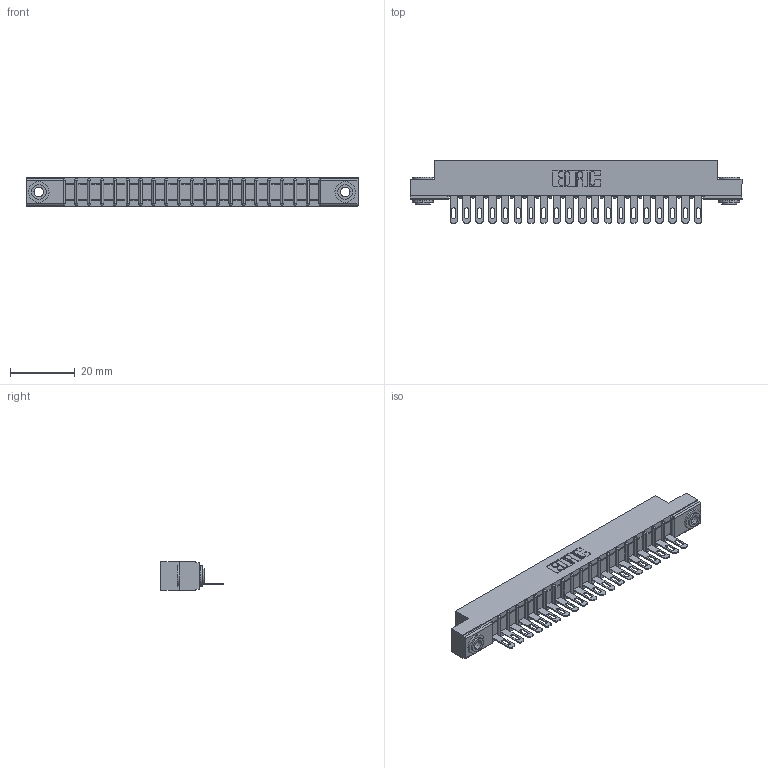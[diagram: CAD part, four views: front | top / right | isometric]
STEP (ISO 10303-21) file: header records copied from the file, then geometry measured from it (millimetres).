
FILE_DESCRIPTION (( 'STEP AP203' ), '1' );
FILE_NAME ('307-020-505-103.STEP', '2019-09-03T18:37:47', ( '' ), ( '' ), 'SwSTEP 2.0', 'SolidWorks 2016', '' );
FILE_SCHEMA (( 'CONFIG_CONTROL_DESIGN' ));
Length unit declared in the file: inch
Products named in the file (4): 345-250-002_345-250-002-102; 307 Part_.156 Dia Mounting Holes; 307-290-001_505; 307-020-505-103
Assembly tree (23 placements, depth 2):
  307-020-505-103
    307 Part_.156 Dia Mounting Holes
    307-290-001_505  x20
    345-250-002_345-250-002-102  x2
Bounding box: 102.26 x 19.18 x 8.71 mm (x, y, z)
Volume: 6489.7 mm3; surface area: 10400.1 mm2
Topology: 23 solids, 23 shells, 1311 faces, 3675 edges, 2362 vertices
Faces by surface type: plane 814, cylinder 447, sphere 42, cone 8
Entity records: 20897 total; most frequent: CARTESIAN_POINT 3489, ORIENTED_EDGE 3466, DIRECTION 3423, EDGE_CURVE 1733, VECTOR 1311, LINE 1311, VERTEX_POINT 1122, AXIS2_PLACEMENT_3D 1056
